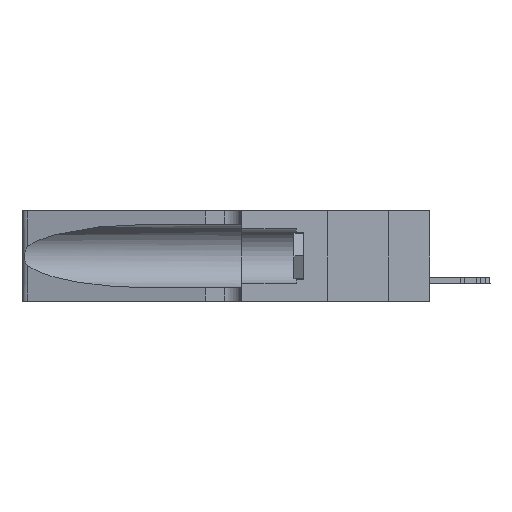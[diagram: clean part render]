
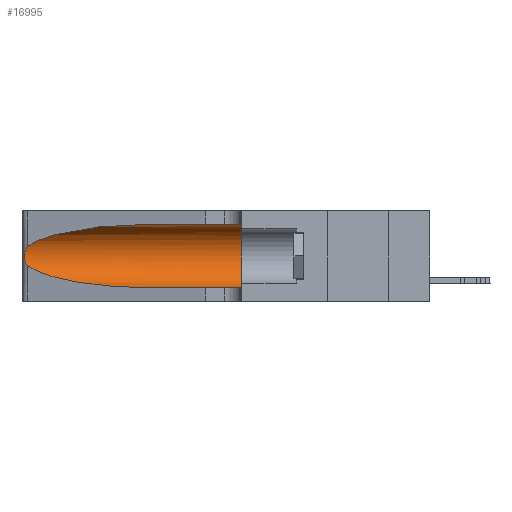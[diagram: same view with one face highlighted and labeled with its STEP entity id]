
A CAD part, left-side view. The second image highlights one B-rep face of the part: STEP entity #16995.
In plain terms, the highlighted cylindrical face has radius 3.308 mm (diameter 6.617 mm), a partial arc.
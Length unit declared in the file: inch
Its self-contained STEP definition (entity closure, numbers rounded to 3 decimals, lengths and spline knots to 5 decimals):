
#580 = VECTOR ( 'NONE', #4342, 39.37008 ) ;
#2395 = VERTEX_POINT ( 'NONE', #4777 ) ;
#2675 = CARTESIAN_POINT ( 'NONE',  ( 0.2373, 1.15595, 0.28018 ) ) ;
#3049 = CARTESIAN_POINT ( 'NONE',  ( 0.25639, 1.23184, 0.21858 ) ) ;
#4342 = DIRECTION ( 'NONE',  ( 0., -1., 0. ) ) ;
#4765 = ORIENTED_EDGE ( 'NONE', *, *, #38726, .T. ) ;
#4777 = CARTESIAN_POINT ( 'NONE',  ( 0.25487, 1.22718, 0.14631 ) ) ;
#6240 = CARTESIAN_POINT ( 'NONE',  ( 0.26018, 1.23835, 0.19895 ) ) ;
#6505 = EDGE_CURVE ( 'NONE', #16613, #6850, #44711, .T. ) ;
#6735 = CARTESIAN_POINT ( 'NONE',  ( 0.25854, 1.2359, 0.20912 ) ) ;
#6850 = VERTEX_POINT ( 'NONE', #35774 ) ;
#7299 = VERTEX_POINT ( 'NONE', #48483 ) ;
#8609 =( BOUNDED_CURVE ( )  B_SPLINE_CURVE ( 3, ( #25045, #10038, #47941, #28711 ),
 .UNSPECIFIED., .F., .F. ) 
 B_SPLINE_CURVE_WITH_KNOTS ( ( 4, 4 ),
 ( 3.44316, 4.71239 ),
 .UNSPECIFIED. ) 
 CURVE ( )  GEOMETRIC_REPRESENTATION_ITEM ( )  RATIONAL_B_SPLINE_CURVE ( ( 1., 0.87, 0.87, 1. ) ) 
 REPRESENTATION_ITEM ( '' )  );
#8884 = AXIS2_PLACEMENT_3D ( 'NONE', #33274, #29944, #22120 ) ;
#10038 = CARTESIAN_POINT ( 'NONE',  ( 0.2373, 1.15595, 0.08982 ) ) ;
#10617 = CARTESIAN_POINT ( 'NONE',  ( 0.25856, 1.23593, 0.16098 ) ) ;
#11479 = CARTESIAN_POINT ( 'NONE',  ( 0.1305, 1.61858, 0.05475 ) ) ;
#11760 =( BOUNDED_CURVE ( )  B_SPLINE_CURVE ( 3, ( #16389, #13037, #2675, #29288 ),
 .UNSPECIFIED., .F., .T. ) 
 B_SPLINE_CURVE_WITH_KNOTS ( ( 4, 4 ),
 ( 1.5708, 2.84003 ),
 .UNSPECIFIED. ) 
 CURVE ( )  GEOMETRIC_REPRESENTATION_ITEM ( )  RATIONAL_B_SPLINE_CURVE ( ( 1., 0.87, 0.87, 1. ) ) 
 REPRESENTATION_ITEM ( '' )  );
#13037 = CARTESIAN_POINT ( 'NONE',  ( 0.18966, 0.96281, 0.31525 ) ) ;
#13613 = ORIENTED_EDGE ( 'NONE', *, *, #49340, .F. ) ;
#15893 = ORIENTED_EDGE ( 'NONE', *, *, #35150, .T. ) ;
#16389 = CARTESIAN_POINT ( 'NONE',  ( 0.1305, 0.72297, 0.31525 ) ) ;
#16613 = VERTEX_POINT ( 'NONE', #36148 ) ;
#16865 = ORIENTED_EDGE ( 'NONE', *, *, #44959, .T. ) ;
#16995 = ADVANCED_FACE ( 'NONE', ( #46644 ), #45487, .F. ) ;
#18008 = CARTESIAN_POINT ( 'NONE',  ( 0.26017, 1.23833, 0.17102 ) ) ;
#18600 = VECTOR ( 'NONE', #23280, 39.37008 ) ;
#19640 = CARTESIAN_POINT ( 'NONE',  ( 0.25487, 1.22718, 0.22369 ) ) ;
#21703 = CARTESIAN_POINT ( 'NONE',  ( 0.25787, 1.23484, 0.2124 ) ) ;
#21872 = CARTESIAN_POINT ( 'NONE',  ( 0.25639, 1.23186, 0.15144 ) ) ;
#22120 = DIRECTION ( 'NONE',  ( 0., 0., -1. ) ) ;
#22961 = DIRECTION ( 'NONE',  ( 0., 1., 0. ) ) ;
#23280 = DIRECTION ( 'NONE',  ( 0., -1., 0. ) ) ;
#23619 = ORIENTED_EDGE ( 'NONE', *, *, #6505, .T. ) ;
#25045 = CARTESIAN_POINT ( 'NONE',  ( 0.25487, 1.22718, 0.14631 ) ) ;
#25618 = CARTESIAN_POINT ( 'NONE',  ( 0.26075, 1.23896, 0.178 ) ) ;
#26139 = CARTESIAN_POINT ( 'NONE',  ( 0.25487, 1.22718, 0.22369 ) ) ;
#27102 = ORIENTED_EDGE ( 'NONE', *, *, #34055, .F. ) ;
#28316 = VERTEX_POINT ( 'NONE', #19640 ) ;
#28711 = CARTESIAN_POINT ( 'NONE',  ( 0.1305, 0.72297, 0.05475 ) ) ;
#28733 = B_SPLINE_CURVE_WITH_KNOTS ( 'NONE', 3,
 ( #26139, #44653, #3049, #21703, #6735, #6240, #33207, #25618, #18008, #10617, #44995, #21872, #30049, #41471 ),
 .UNSPECIFIED., .F., .F.,
 ( 4, 2, 2, 2, 2, 2, 4 ),
 ( 0., 0.00027, 0.00053, 0.00107, 0.0016, 0.00187, 0.00214 ),
 .UNSPECIFIED. ) ;
#28811 = LINE ( 'NONE', #47502, #18600 ) ;
#29026 = AXIS2_PLACEMENT_3D ( 'NONE', #40466, #22961, #30835 ) ;
#29288 = CARTESIAN_POINT ( 'NONE',  ( 0.25487, 1.22718, 0.22369 ) ) ;
#29944 = DIRECTION ( 'NONE',  ( 0., -1., 0. ) ) ;
#30049 = CARTESIAN_POINT ( 'NONE',  ( 0.25555, 1.22993, 0.14849 ) ) ;
#30835 = DIRECTION ( 'NONE',  ( 0., 0., 1. ) ) ;
#33072 = CARTESIAN_POINT ( 'NONE',  ( 0.1305, 0.72297, 0.31525 ) ) ;
#33207 = CARTESIAN_POINT ( 'NONE',  ( 0.26075, 1.23896, 0.19203 ) ) ;
#33274 = CARTESIAN_POINT ( 'NONE',  ( 0.1305, 1.61858, 0.185 ) ) ;
#34055 = EDGE_CURVE ( 'NONE', #7299, #6850, #34776, .T. ) ;
#34776 = CIRCLE ( 'NONE', #29026, 0.13025 ) ;
#35150 = EDGE_CURVE ( 'NONE', #46083, #28316, #11760, .T. ) ;
#35774 = CARTESIAN_POINT ( 'NONE',  ( 0.1305, 0.35, 0.05475 ) ) ;
#36148 = CARTESIAN_POINT ( 'NONE',  ( 0.1305, 0.72297, 0.05475 ) ) ;
#38726 = EDGE_CURVE ( 'NONE', #28316, #2395, #28733, .T. ) ;
#40466 = CARTESIAN_POINT ( 'NONE',  ( 0.1305, 0.35, 0.185 ) ) ;
#40700 = EDGE_LOOP ( 'NONE', ( #15893, #4765, #16865, #23619, #27102, #13613 ) ) ;
#41471 = CARTESIAN_POINT ( 'NONE',  ( 0.25487, 1.22718, 0.14631 ) ) ;
#44653 = CARTESIAN_POINT ( 'NONE',  ( 0.25555, 1.22994, 0.2215 ) ) ;
#44711 = LINE ( 'NONE', #11479, #580 ) ;
#44959 = EDGE_CURVE ( 'NONE', #2395, #16613, #8609, .T. ) ;
#44995 = CARTESIAN_POINT ( 'NONE',  ( 0.25789, 1.23486, 0.15765 ) ) ;
#45487 = CYLINDRICAL_SURFACE ( 'NONE', #8884, 0.13025 ) ;
#46083 = VERTEX_POINT ( 'NONE', #33072 ) ;
#46644 = FACE_OUTER_BOUND ( 'NONE', #40700, .T. ) ;
#47502 = CARTESIAN_POINT ( 'NONE',  ( 0.1305, 1.61858, 0.31525 ) ) ;
#47941 = CARTESIAN_POINT ( 'NONE',  ( 0.18966, 0.96281, 0.05475 ) ) ;
#48483 = CARTESIAN_POINT ( 'NONE',  ( 0.1305, 0.35, 0.31525 ) ) ;
#49340 = EDGE_CURVE ( 'NONE', #46083, #7299, #28811, .T. ) ;
